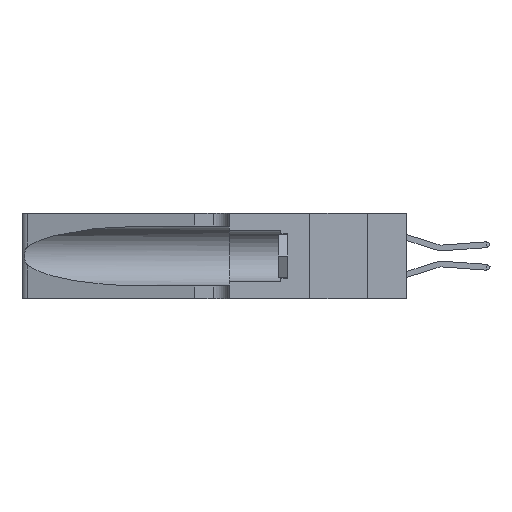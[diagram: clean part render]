
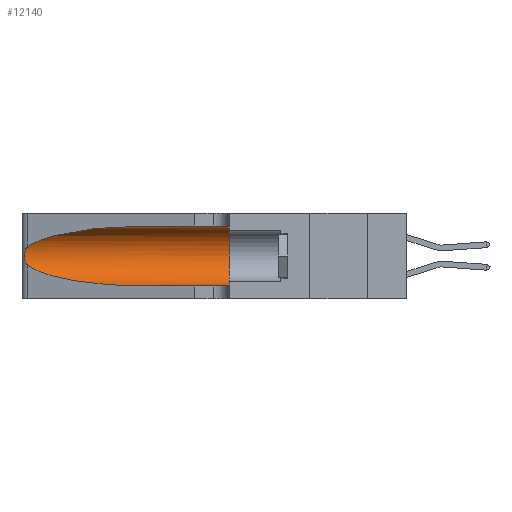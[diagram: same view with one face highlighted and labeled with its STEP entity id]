
A CAD part, left-side view. The second image highlights one B-rep face of the part: STEP entity #12140.
In plain terms, the highlighted cylindrical face has radius 3.308 mm (diameter 6.617 mm), a partial arc.
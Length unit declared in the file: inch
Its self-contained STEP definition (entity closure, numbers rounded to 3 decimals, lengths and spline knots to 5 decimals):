
#407 = DIRECTION ( 'NONE',  ( 0., -1., 0. ) ) ;
#432 = CARTESIAN_POINT ( 'NONE',  ( 0.25856, 1.23593, 0.16098 ) ) ;
#1324 = CARTESIAN_POINT ( 'NONE',  ( 0.25487, 1.22718, 0.22369 ) ) ;
#2047 = VECTOR ( 'NONE', #12328, 39.37008 ) ;
#2931 = VERTEX_POINT ( 'NONE', #13522 ) ;
#3321 = CARTESIAN_POINT ( 'NONE',  ( 0.18966, 0.96281, 0.31525 ) ) ;
#3513 = CARTESIAN_POINT ( 'NONE',  ( 0.2373, 1.15595, 0.28018 ) ) ;
#4264 = CARTESIAN_POINT ( 'NONE',  ( 0.25487, 1.22718, 0.14631 ) ) ;
#4598 = CARTESIAN_POINT ( 'NONE',  ( 0.25487, 1.22718, 0.14631 ) ) ;
#5306 = AXIS2_PLACEMENT_3D ( 'NONE', #15574, #407, #19903 ) ;
#5426 = CARTESIAN_POINT ( 'NONE',  ( 0.25639, 1.23184, 0.21858 ) ) ;
#6360 = CARTESIAN_POINT ( 'NONE',  ( 0.26018, 1.23835, 0.19895 ) ) ;
#6387 = CARTESIAN_POINT ( 'NONE',  ( 0.1305, 0.72297, 0.05475 ) ) ;
#6453 = CARTESIAN_POINT ( 'NONE',  ( 0.26075, 1.23896, 0.178 ) ) ;
#7148 = DIRECTION ( 'NONE',  ( 0., 1., 0. ) ) ;
#7776 = ORIENTED_EDGE ( 'NONE', *, *, #20248, .F. ) ;
#7977 = B_SPLINE_CURVE_WITH_KNOTS ( 'NONE', 3,
 ( #9645, #10016, #5426, #22932, #8699, #6360, #25666, #6453, #15064, #432, #17655, #17296, #19483, #4598 ),
 .UNSPECIFIED., .F., .F.,
 ( 4, 2, 2, 2, 2, 2, 4 ),
 ( 0., 0.00027, 0.00053, 0.00107, 0.0016, 0.00187, 0.00214 ),
 .UNSPECIFIED. ) ;
#8115 = CARTESIAN_POINT ( 'NONE',  ( 0.1305, 1.61858, 0.05475 ) ) ;
#8158 = CARTESIAN_POINT ( 'NONE',  ( 0.1305, 1.61858, 0.31525 ) ) ;
#8699 = CARTESIAN_POINT ( 'NONE',  ( 0.25854, 1.2359, 0.20912 ) ) ;
#8804 = LINE ( 'NONE', #8158, #10163 ) ;
#9631 = CARTESIAN_POINT ( 'NONE',  ( 0.1305, 0.35, 0.31525 ) ) ;
#9645 = CARTESIAN_POINT ( 'NONE',  ( 0.25487, 1.22718, 0.22369 ) ) ;
#9894 = VERTEX_POINT ( 'NONE', #1324 ) ;
#10016 = CARTESIAN_POINT ( 'NONE',  ( 0.25555, 1.22994, 0.2215 ) ) ;
#10163 = VECTOR ( 'NONE', #25934, 39.37008 ) ;
#10714 = LINE ( 'NONE', #8115, #2047 ) ;
#11442 = CARTESIAN_POINT ( 'NONE',  ( 0.1305, 0.72297, 0.31525 ) ) ;
#11466 = EDGE_CURVE ( 'NONE', #9894, #2931, #7977, .T. ) ;
#11888 = CARTESIAN_POINT ( 'NONE',  ( 0.1305, 0.72297, 0.31525 ) ) ;
#12140 = ADVANCED_FACE ( 'NONE', ( #25993 ), #13690, .F. ) ;
#12328 = DIRECTION ( 'NONE',  ( 0., -1., 0. ) ) ;
#13190 = ORIENTED_EDGE ( 'NONE', *, *, #20678, .T. ) ;
#13251 =( BOUNDED_CURVE ( )  B_SPLINE_CURVE ( 3, ( #11888, #3321, #3513, #18413 ),
 .UNSPECIFIED., .F., .T. ) 
 B_SPLINE_CURVE_WITH_KNOTS ( ( 4, 4 ),
 ( 1.5708, 2.84003 ),
 .UNSPECIFIED. ) 
 CURVE ( )  GEOMETRIC_REPRESENTATION_ITEM ( )  RATIONAL_B_SPLINE_CURVE ( ( 1., 0.87, 0.87, 1. ) ) 
 REPRESENTATION_ITEM ( '' )  );
#13412 = CIRCLE ( 'NONE', #26678, 0.13025 ) ;
#13522 = CARTESIAN_POINT ( 'NONE',  ( 0.25487, 1.22718, 0.14631 ) ) ;
#13690 = CYLINDRICAL_SURFACE ( 'NONE', #5306, 0.13025 ) ;
#14516 = VERTEX_POINT ( 'NONE', #11442 ) ;
#14986 = CARTESIAN_POINT ( 'NONE',  ( 0.2373, 1.15595, 0.08982 ) ) ;
#15064 = CARTESIAN_POINT ( 'NONE',  ( 0.26017, 1.23833, 0.17102 ) ) ;
#15574 = CARTESIAN_POINT ( 'NONE',  ( 0.1305, 1.61858, 0.185 ) ) ;
#15738 = ORIENTED_EDGE ( 'NONE', *, *, #18028, .T. ) ;
#16783 = CARTESIAN_POINT ( 'NONE',  ( 0.18966, 0.96281, 0.05475 ) ) ;
#17296 = CARTESIAN_POINT ( 'NONE',  ( 0.25639, 1.23186, 0.15144 ) ) ;
#17530 = ORIENTED_EDGE ( 'NONE', *, *, #18567, .F. ) ;
#17640 = CARTESIAN_POINT ( 'NONE',  ( 0.1305, 0.35, 0.05475 ) ) ;
#17655 = CARTESIAN_POINT ( 'NONE',  ( 0.25789, 1.23486, 0.15765 ) ) ;
#18006 = CARTESIAN_POINT ( 'NONE',  ( 0.1305, 0.35, 0.185 ) ) ;
#18028 = EDGE_CURVE ( 'NONE', #2931, #20783, #23533, .T. ) ;
#18413 = CARTESIAN_POINT ( 'NONE',  ( 0.25487, 1.22718, 0.22369 ) ) ;
#18567 = EDGE_CURVE ( 'NONE', #19095, #25965, #13412, .T. ) ;
#19095 = VERTEX_POINT ( 'NONE', #9631 ) ;
#19483 = CARTESIAN_POINT ( 'NONE',  ( 0.25555, 1.22993, 0.14849 ) ) ;
#19903 = DIRECTION ( 'NONE',  ( 0., 0., -1. ) ) ;
#20248 = EDGE_CURVE ( 'NONE', #14516, #19095, #8804, .T. ) ;
#20678 = EDGE_CURVE ( 'NONE', #14516, #9894, #13251, .T. ) ;
#20783 = VERTEX_POINT ( 'NONE', #20791 ) ;
#20791 = CARTESIAN_POINT ( 'NONE',  ( 0.1305, 0.72297, 0.05475 ) ) ;
#21158 = ORIENTED_EDGE ( 'NONE', *, *, #11466, .T. ) ;
#21382 = ORIENTED_EDGE ( 'NONE', *, *, #26219, .T. ) ;
#22016 = EDGE_LOOP ( 'NONE', ( #13190, #21158, #15738, #21382, #17530, #7776 ) ) ;
#22932 = CARTESIAN_POINT ( 'NONE',  ( 0.25787, 1.23484, 0.2124 ) ) ;
#23533 =( BOUNDED_CURVE ( )  B_SPLINE_CURVE ( 3, ( #4264, #14986, #16783, #6387 ),
 .UNSPECIFIED., .F., .T. ) 
 B_SPLINE_CURVE_WITH_KNOTS ( ( 4, 4 ),
 ( 3.44316, 4.71239 ),
 .UNSPECIFIED. ) 
 CURVE ( )  GEOMETRIC_REPRESENTATION_ITEM ( )  RATIONAL_B_SPLINE_CURVE ( ( 1., 0.87, 0.87, 1. ) ) 
 REPRESENTATION_ITEM ( '' )  );
#25666 = CARTESIAN_POINT ( 'NONE',  ( 0.26075, 1.23896, 0.19203 ) ) ;
#25934 = DIRECTION ( 'NONE',  ( 0., -1., 0. ) ) ;
#25965 = VERTEX_POINT ( 'NONE', #17640 ) ;
#25993 = FACE_OUTER_BOUND ( 'NONE', #22016, .T. ) ;
#26219 = EDGE_CURVE ( 'NONE', #20783, #25965, #10714, .T. ) ;
#26531 = DIRECTION ( 'NONE',  ( 0., 0., 1. ) ) ;
#26678 = AXIS2_PLACEMENT_3D ( 'NONE', #18006, #7148, #26531 ) ;
